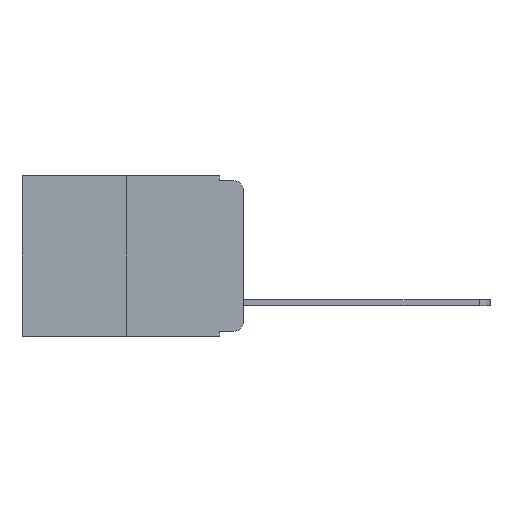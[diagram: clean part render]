
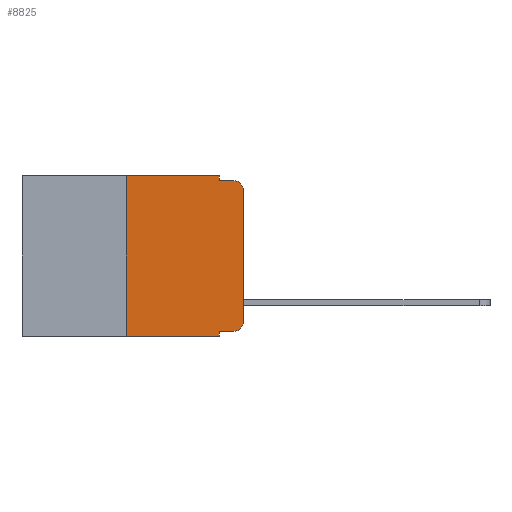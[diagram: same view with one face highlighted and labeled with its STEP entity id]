
A CAD part, left-side view. The second image highlights one B-rep face of the part: STEP entity #8825.
In plain terms, the highlighted planar face has unit normal (-1, 0, 0).
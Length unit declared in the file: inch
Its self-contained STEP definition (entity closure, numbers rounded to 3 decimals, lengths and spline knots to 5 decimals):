
#89 = CARTESIAN_POINT ( 'NONE',  ( 0., 0.02, -0.313 ) ) ;
#97 = DIRECTION ( 'NONE',  ( 0., -1., 0. ) ) ;
#128 = CARTESIAN_POINT ( 'NONE',  ( 0., 0.25, 0. ) ) ;
#258 = DIRECTION ( 'NONE',  ( -1., 0., 0. ) ) ;
#305 = LINE ( 'NONE', #3182, #10585 ) ;
#468 = LINE ( 'NONE', #7066, #2343 ) ;
#653 = ORIENTED_EDGE ( 'NONE', *, *, #6143, .T. ) ;
#764 = EDGE_LOOP ( 'NONE', ( #6004, #1259, #958, #3426, #1766, #1369, #1196, #847, #1396, #653 ) ) ;
#763 = VECTOR ( 'NONE', #10455, 39.37008 ) ;
#767 = CARTESIAN_POINT ( 'NONE',  ( 0., 0.051, -0.01 ) ) ;
#788 = VECTOR ( 'NONE', #97, 39.37008 ) ;
#847 = ORIENTED_EDGE ( 'NONE', *, *, #6170, .F. ) ;
#855 = CARTESIAN_POINT ( 'NONE',  ( 0., 0.25, -0.343 ) ) ;
#958 = ORIENTED_EDGE ( 'NONE', *, *, #6446, .F. ) ;
#1081 = DIRECTION ( 'NONE',  ( 0., 0., -1. ) ) ;
#1196 = ORIENTED_EDGE ( 'NONE', *, *, #5157, .T. ) ;
#1259 = ORIENTED_EDGE ( 'NONE', *, *, #6211, .T. ) ;
#1369 = ORIENTED_EDGE ( 'NONE', *, *, #6184, .F. ) ;
#1396 = ORIENTED_EDGE ( 'NONE', *, *, #6174, .T. ) ;
#1480 = AXIS2_PLACEMENT_3D ( 'NONE', #5590, #258, #6408 ) ;
#1540 = AXIS2_PLACEMENT_3D ( 'NONE', #89, #6266, #1081 ) ;
#1684 = CARTESIAN_POINT ( 'NONE',  ( 0., 0.051, -0.343 ) ) ;
#1766 = ORIENTED_EDGE ( 'NONE', *, *, #8684, .F. ) ;
#1876 = CARTESIAN_POINT ( 'NONE',  ( 0., 0.051, 0. ) ) ;
#2027 = VERTEX_POINT ( 'NONE', #855 ) ;
#2050 = VERTEX_POINT ( 'NONE', #7217 ) ;
#2090 = VECTOR ( 'NONE', #5030, 39.37008 ) ;
#2161 = CARTESIAN_POINT ( 'NONE',  ( 0., 0.02, -0.333 ) ) ;
#2343 = VECTOR ( 'NONE', #6298, 39.37008 ) ;
#2785 = DIRECTION ( 'NONE',  ( 0., 0., -1. ) ) ;
#2916 = CIRCLE ( 'NONE', #1540, 0.02 ) ;
#3167 = LINE ( 'NONE', #767, #763 ) ;
#3182 = CARTESIAN_POINT ( 'NONE',  ( 0., 0., 0. ) ) ;
#3426 = ORIENTED_EDGE ( 'NONE', *, *, #6101, .F. ) ;
#3647 = VERTEX_POINT ( 'NONE', #3764 ) ;
#3764 = CARTESIAN_POINT ( 'NONE',  ( 0., 0.051, -0.333 ) ) ;
#3833 = LINE ( 'NONE', #1876, #7839 ) ;
#3937 = AXIS2_PLACEMENT_3D ( 'NONE', #4927, #10247, #5738 ) ;
#4030 = PLANE ( 'NONE',  #3937 ) ;
#4392 = VERTEX_POINT ( 'NONE', #1684 ) ;
#4415 = LINE ( 'NONE', #128, #8406 ) ;
#4595 = VERTEX_POINT ( 'NONE', #9265 ) ;
#4623 = CARTESIAN_POINT ( 'NONE',  ( 0., 0.473, 0. ) ) ;
#4691 = DIRECTION ( 'NONE',  ( 0., -1., 0. ) ) ;
#4797 = VERTEX_POINT ( 'NONE', #7801 ) ;
#4927 = CARTESIAN_POINT ( 'NONE',  ( 0., 0.473, 0. ) ) ;
#5018 = CARTESIAN_POINT ( 'NONE',  ( 0., 0.473, -0.343 ) ) ;
#5030 = DIRECTION ( 'NONE',  ( 0., -1., 0. ) ) ;
#5157 = EDGE_CURVE ( 'NONE', #2027, #4392, #5877, .T. ) ;
#5590 = CARTESIAN_POINT ( 'NONE',  ( 0., 0.02, -0.03 ) ) ;
#5701 = VERTEX_POINT ( 'NONE', #6311 ) ;
#5738 = DIRECTION ( 'NONE',  ( 0., 0., -1. ) ) ;
#5877 = LINE ( 'NONE', #5018, #2090 ) ;
#6004 = ORIENTED_EDGE ( 'NONE', *, *, #6310, .T. ) ;
#6101 = EDGE_CURVE ( 'NONE', #5701, #4797, #3833, .T. ) ;
#6143 = EDGE_CURVE ( 'NONE', #8375, #4595, #2916, .T. ) ;
#6170 = EDGE_CURVE ( 'NONE', #3647, #4392, #468, .T. ) ;
#6174 = EDGE_CURVE ( 'NONE', #3647, #8375, #8635, .T. ) ;
#6184 = EDGE_CURVE ( 'NONE', #2027, #8726, #4415, .T. ) ;
#6211 = EDGE_CURVE ( 'NONE', #2050, #10218, #8179, .T. ) ;
#6266 = DIRECTION ( 'NONE',  ( -1., 0., 0. ) ) ;
#6298 = DIRECTION ( 'NONE',  ( 0., 0., -1. ) ) ;
#6310 = EDGE_CURVE ( 'NONE', #4595, #2050, #305, .T. ) ;
#6311 = CARTESIAN_POINT ( 'NONE',  ( 0., 0.051, 0. ) ) ;
#6408 = DIRECTION ( 'NONE',  ( 0., 0., -1. ) ) ;
#6446 = EDGE_CURVE ( 'NONE', #4797, #10218, #3167, .T. ) ;
#7066 = CARTESIAN_POINT ( 'NONE',  ( 0., 0.051, 0. ) ) ;
#7142 = CARTESIAN_POINT ( 'NONE',  ( 0., 0.25, 0. ) ) ;
#7217 = CARTESIAN_POINT ( 'NONE',  ( 0., 0., -0.03 ) ) ;
#7373 = DIRECTION ( 'NONE',  ( 0., 0., 1. ) ) ;
#7801 = CARTESIAN_POINT ( 'NONE',  ( 0., 0.051, -0.01 ) ) ;
#7839 = VECTOR ( 'NONE', #2785, 39.37008 ) ;
#8179 = CIRCLE ( 'NONE', #1480, 0.02 ) ;
#8375 = VERTEX_POINT ( 'NONE', #2161 ) ;
#8406 = VECTOR ( 'NONE', #8650, 39.37008 ) ;
#8422 = CARTESIAN_POINT ( 'NONE',  ( 0., 0.02, -0.01 ) ) ;
#8635 = LINE ( 'NONE', #9347, #10498 ) ;
#8650 = DIRECTION ( 'NONE',  ( 0., 0., 1. ) ) ;
#8684 = EDGE_CURVE ( 'NONE', #8726, #5701, #9562, .T. ) ;
#8726 = VERTEX_POINT ( 'NONE', #7142 ) ;
#8825 = ADVANCED_FACE ( 'NONE', ( #8978 ), #4030, .F. ) ;
#8978 = FACE_OUTER_BOUND ( 'NONE', #764, .T. ) ;
#9265 = CARTESIAN_POINT ( 'NONE',  ( 0., 0., -0.313 ) ) ;
#9347 = CARTESIAN_POINT ( 'NONE',  ( 0., 0.051, -0.333 ) ) ;
#9562 = LINE ( 'NONE', #4623, #788 ) ;
#10218 = VERTEX_POINT ( 'NONE', #8422 ) ;
#10247 = DIRECTION ( 'NONE',  ( 1., 0., 0. ) ) ;
#10455 = DIRECTION ( 'NONE',  ( 0., -1., 0. ) ) ;
#10498 = VECTOR ( 'NONE', #4691, 39.37008 ) ;
#10585 = VECTOR ( 'NONE', #7373, 39.37008 ) ;
